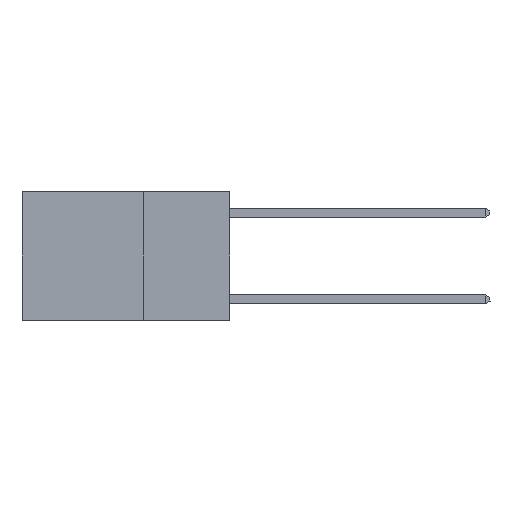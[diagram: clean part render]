
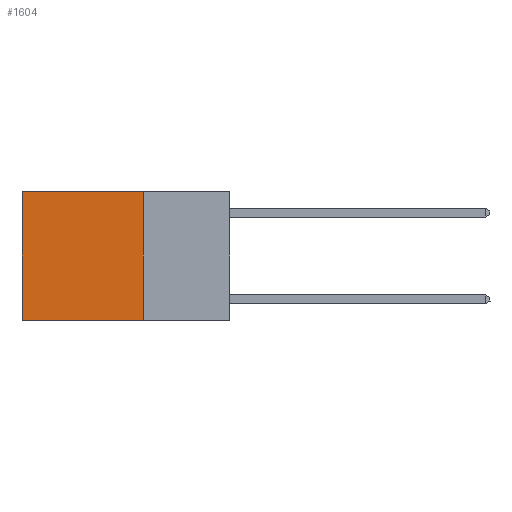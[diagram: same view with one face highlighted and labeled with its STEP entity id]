
A CAD part, left-side view. The second image highlights one B-rep face of the part: STEP entity #1604.
In plain terms, the highlighted planar face has unit normal (-1, 0, 0).
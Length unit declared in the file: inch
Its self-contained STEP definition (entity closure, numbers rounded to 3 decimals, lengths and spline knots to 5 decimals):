
#426 = AXIS2_PLACEMENT_3D ( 'NONE', #2225, #11228, #5423 ) ;
#1564 = VERTEX_POINT ( 'NONE', #6457 ) ;
#1604 = ADVANCED_FACE ( 'NONE', ( #4183 ), #4336, .F. ) ;
#2128 = ORIENTED_EDGE ( 'NONE', *, *, #11262, .T. ) ;
#2225 = CARTESIAN_POINT ( 'NONE',  ( 0.2625, 0.25, 0. ) ) ;
#2319 = EDGE_CURVE ( 'NONE', #11426, #7117, #10816, .T. ) ;
#3067 = VECTOR ( 'NONE', #8000, 39.37008 ) ;
#3459 = CARTESIAN_POINT ( 'NONE',  ( 0.2625, 0.25, 0. ) ) ;
#3482 = VECTOR ( 'NONE', #12363, 39.37008 ) ;
#3558 = CARTESIAN_POINT ( 'NONE',  ( 0.2625, 0.6, -0.37 ) ) ;
#3604 = CARTESIAN_POINT ( 'NONE',  ( 0.2625, 0.6, 0. ) ) ;
#3788 = CARTESIAN_POINT ( 'NONE',  ( 0.2625, 0.25, -0.37 ) ) ;
#4183 = FACE_OUTER_BOUND ( 'NONE', #8715, .T. ) ;
#4336 = PLANE ( 'NONE',  #426 ) ;
#4482 = CARTESIAN_POINT ( 'NONE',  ( 0.2625, 0.25, 0. ) ) ;
#5069 = VECTOR ( 'NONE', #7687, 39.37008 ) ;
#5251 = ORIENTED_EDGE ( 'NONE', *, *, #10558, .F. ) ;
#5423 = DIRECTION ( 'NONE',  ( 0., 0., -1. ) ) ;
#6457 = CARTESIAN_POINT ( 'NONE',  ( 0.2625, 0.25, -0.37 ) ) ;
#6819 = CARTESIAN_POINT ( 'NONE',  ( 0.2625, 0.6, 0. ) ) ;
#6931 = CARTESIAN_POINT ( 'NONE',  ( 0.2625, 0.25, 0. ) ) ;
#7117 = VERTEX_POINT ( 'NONE', #3558 ) ;
#7199 = EDGE_CURVE ( 'NONE', #8323, #1564, #9244, .T. ) ;
#7687 = DIRECTION ( 'NONE',  ( 0., 1., 0. ) ) ;
#8000 = DIRECTION ( 'NONE',  ( 0., 1., 0. ) ) ;
#8026 = ORIENTED_EDGE ( 'NONE', *, *, #2319, .T. ) ;
#8323 = VERTEX_POINT ( 'NONE', #3459 ) ;
#8715 = EDGE_LOOP ( 'NONE', ( #8026, #5251, #9581, #2128 ) ) ;
#9244 = LINE ( 'NONE', #6931, #10791 ) ;
#9581 = ORIENTED_EDGE ( 'NONE', *, *, #7199, .F. ) ;
#10301 = LINE ( 'NONE', #4482, #5069 ) ;
#10558 = EDGE_CURVE ( 'NONE', #1564, #7117, #11018, .T. ) ;
#10791 = VECTOR ( 'NONE', #12479, 39.37008 ) ;
#10816 = LINE ( 'NONE', #3604, #3482 ) ;
#11018 = LINE ( 'NONE', #3788, #3067 ) ;
#11228 = DIRECTION ( 'NONE',  ( 1., 0., 0. ) ) ;
#11262 = EDGE_CURVE ( 'NONE', #8323, #11426, #10301, .T. ) ;
#11426 = VERTEX_POINT ( 'NONE', #6819 ) ;
#12363 = DIRECTION ( 'NONE',  ( 0., 0., -1. ) ) ;
#12479 = DIRECTION ( 'NONE',  ( 0., 0., -1. ) ) ;
